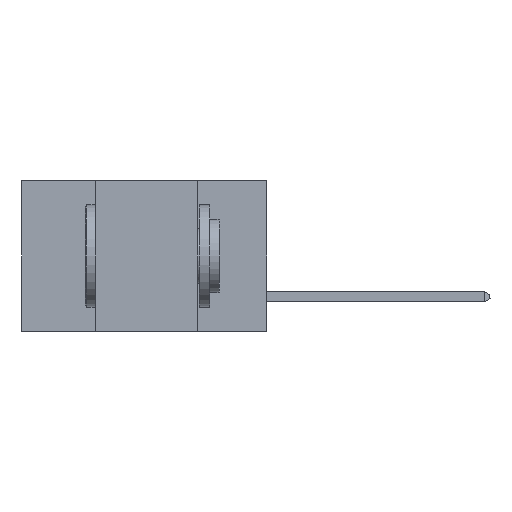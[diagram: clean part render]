
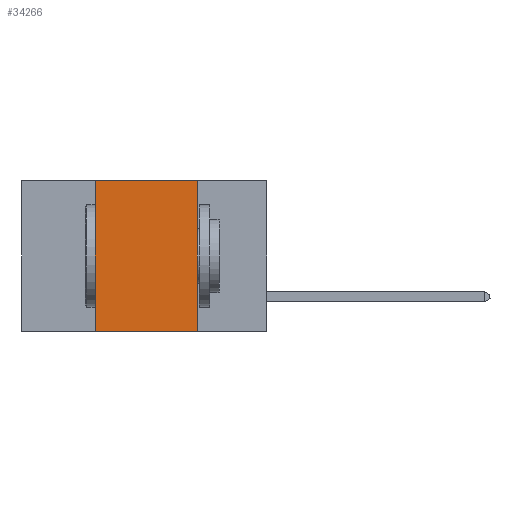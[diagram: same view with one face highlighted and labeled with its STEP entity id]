
A CAD part, left-side view. The second image highlights one B-rep face of the part: STEP entity #34266.
In plain terms, the highlighted planar face has unit normal (-1, 0, 0).
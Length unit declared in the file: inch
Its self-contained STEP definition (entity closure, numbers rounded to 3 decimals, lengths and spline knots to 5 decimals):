
#4189 = FACE_OUTER_BOUND ( 'NONE', #28316, .T. ) ;
#5034 = VERTEX_POINT ( 'NONE', #29297 ) ;
#5312 = CARTESIAN_POINT ( 'NONE',  ( 0., 0.17, 0. ) ) ;
#5532 = DIRECTION ( 'NONE',  ( 1., 0., 0. ) ) ;
#5768 = VERTEX_POINT ( 'NONE', #13067 ) ;
#5872 = PLANE ( 'NONE',  #11915 ) ;
#6540 = VECTOR ( 'NONE', #29191, 39.37008 ) ;
#6582 = LINE ( 'NONE', #26511, #6540 ) ;
#7029 = ORIENTED_EDGE ( 'NONE', *, *, #17832, .T. ) ;
#7392 = VECTOR ( 'NONE', #13758, 39.37008 ) ;
#11915 = AXIS2_PLACEMENT_3D ( 'NONE', #13751, #5532, #24789 ) ;
#12512 = EDGE_CURVE ( 'NONE', #34841, #5768, #12637, .T. ) ;
#12637 = LINE ( 'NONE', #33163, #21138 ) ;
#13067 = CARTESIAN_POINT ( 'NONE',  ( 0., 0.42, 0. ) ) ;
#13751 = CARTESIAN_POINT ( 'NONE',  ( 0., 0.6, 0. ) ) ;
#13758 = DIRECTION ( 'NONE',  ( 0., -1., 0. ) ) ;
#14398 = ORIENTED_EDGE ( 'NONE', *, *, #12512, .F. ) ;
#14535 = VERTEX_POINT ( 'NONE', #5312 ) ;
#14537 = LINE ( 'NONE', #16696, #7392 ) ;
#15777 = VECTOR ( 'NONE', #17394, 39.37008 ) ;
#16696 = CARTESIAN_POINT ( 'NONE',  ( 0., 0.6, 0. ) ) ;
#17394 = DIRECTION ( 'NONE',  ( 0., 0., -1. ) ) ;
#17724 = EDGE_CURVE ( 'NONE', #5768, #14535, #14537, .T. ) ;
#17832 = EDGE_CURVE ( 'NONE', #34841, #5034, #6582, .T. ) ;
#18449 = ORIENTED_EDGE ( 'NONE', *, *, #24022, .F. ) ;
#19494 = ORIENTED_EDGE ( 'NONE', *, *, #17724, .F. ) ;
#20012 = CARTESIAN_POINT ( 'NONE',  ( 0., 0.17, 0. ) ) ;
#20432 = DIRECTION ( 'NONE',  ( 0., 0., 1. ) ) ;
#21138 = VECTOR ( 'NONE', #20432, 39.37008 ) ;
#24022 = EDGE_CURVE ( 'NONE', #14535, #5034, #30154, .T. ) ;
#24789 = DIRECTION ( 'NONE',  ( 0., 0., -1. ) ) ;
#26511 = CARTESIAN_POINT ( 'NONE',  ( 0., 0.6, -0.37 ) ) ;
#26896 = CARTESIAN_POINT ( 'NONE',  ( 0., 0.42, -0.37 ) ) ;
#28316 = EDGE_LOOP ( 'NONE', ( #18449, #19494, #14398, #7029 ) ) ;
#29191 = DIRECTION ( 'NONE',  ( 0., -1., 0. ) ) ;
#29297 = CARTESIAN_POINT ( 'NONE',  ( 0., 0.17, -0.37 ) ) ;
#30154 = LINE ( 'NONE', #20012, #15777 ) ;
#33163 = CARTESIAN_POINT ( 'NONE',  ( 0., 0.42, 0. ) ) ;
#34266 = ADVANCED_FACE ( 'NONE', ( #4189 ), #5872, .F. ) ;
#34841 = VERTEX_POINT ( 'NONE', #26896 ) ;
